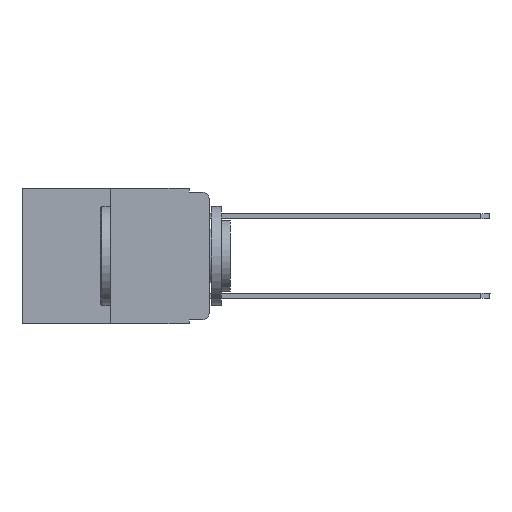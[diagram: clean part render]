
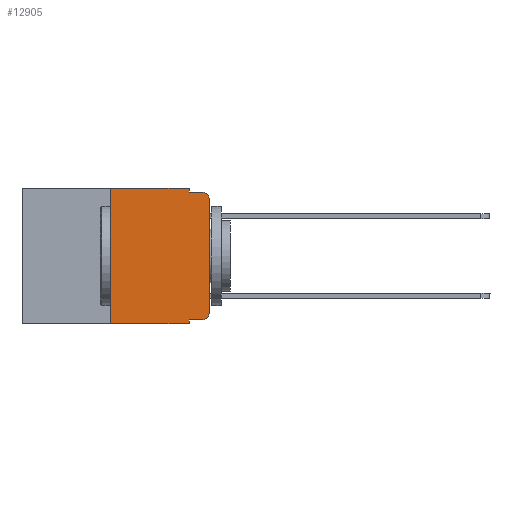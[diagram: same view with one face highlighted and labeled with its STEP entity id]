
A CAD part, left-side view. The second image highlights one B-rep face of the part: STEP entity #12905.
In plain terms, the highlighted planar face has unit normal (-1, 0, 0).
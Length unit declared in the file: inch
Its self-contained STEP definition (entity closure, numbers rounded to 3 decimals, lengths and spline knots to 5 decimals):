
#204 = EDGE_CURVE ( 'NONE', #982, #920, #10719, .T. ) ;
#290 = EDGE_LOOP ( 'NONE', ( #4359, #3330, #5426, #5136, #3894, #4360, #1406, #1857, #1228, #7725 ) ) ;
#349 = VERTEX_POINT ( 'NONE', #13905 ) ;
#687 = DIRECTION ( 'NONE',  ( 1., 0., 0. ) ) ;
#813 = CARTESIAN_POINT ( 'NONE',  ( 0., 0.25, -0.343 ) ) ;
#920 = VERTEX_POINT ( 'NONE', #3082 ) ;
#922 = CARTESIAN_POINT ( 'NONE',  ( 0., 0.051, -0.01 ) ) ;
#982 = VERTEX_POINT ( 'NONE', #15471 ) ;
#996 = DIRECTION ( 'NONE',  ( 0., -1., 0. ) ) ;
#1006 = AXIS2_PLACEMENT_3D ( 'NONE', #8382, #5728, #10912 ) ;
#1228 = ORIENTED_EDGE ( 'NONE', *, *, #2395, .T. ) ;
#1406 = ORIENTED_EDGE ( 'NONE', *, *, #11812, .T. ) ;
#1734 = VERTEX_POINT ( 'NONE', #813 ) ;
#1857 = ORIENTED_EDGE ( 'NONE', *, *, #8401, .F. ) ;
#1917 = CARTESIAN_POINT ( 'NONE',  ( 0., 0.473, 0. ) ) ;
#2174 = CARTESIAN_POINT ( 'NONE',  ( 0., 0.051, -0.333 ) ) ;
#2182 = VECTOR ( 'NONE', #8756, 39.37008 ) ;
#2395 = EDGE_CURVE ( 'NONE', #9739, #3634, #14970, .T. ) ;
#2434 = DIRECTION ( 'NONE',  ( 0., -1., 0. ) ) ;
#2704 = VECTOR ( 'NONE', #2434, 39.37008 ) ;
#3082 = CARTESIAN_POINT ( 'NONE',  ( 0., 0.02, -0.01 ) ) ;
#3330 = ORIENTED_EDGE ( 'NONE', *, *, #204, .T. ) ;
#3525 = DIRECTION ( 'NONE',  ( 0., 0., -1. ) ) ;
#3634 = VERTEX_POINT ( 'NONE', #9755 ) ;
#3663 = CARTESIAN_POINT ( 'NONE',  ( 0., 0.473, -0.343 ) ) ;
#3700 = VECTOR ( 'NONE', #8622, 39.37008 ) ;
#3894 = ORIENTED_EDGE ( 'NONE', *, *, #5141, .F. ) ;
#4005 = DIRECTION ( 'NONE',  ( 0., 0., 1. ) ) ;
#4032 = VERTEX_POINT ( 'NONE', #10787 ) ;
#4270 = PLANE ( 'NONE',  #15746 ) ;
#4359 = ORIENTED_EDGE ( 'NONE', *, *, #12126, .T. ) ;
#4360 = ORIENTED_EDGE ( 'NONE', *, *, #16008, .F. ) ;
#4501 = VERTEX_POINT ( 'NONE', #8149 ) ;
#4517 = DIRECTION ( 'NONE',  ( 0., 0., -1. ) ) ;
#4555 = EDGE_CURVE ( 'NONE', #4501, #4032, #8554, .T. ) ;
#4650 = EDGE_CURVE ( 'NONE', #4032, #920, #6062, .T. ) ;
#4674 = DIRECTION ( 'NONE',  ( 0., 0., -1. ) ) ;
#5136 = ORIENTED_EDGE ( 'NONE', *, *, #4555, .F. ) ;
#5141 = EDGE_CURVE ( 'NONE', #5950, #4501, #9904, .T. ) ;
#5426 = ORIENTED_EDGE ( 'NONE', *, *, #4650, .F. ) ;
#5534 = VECTOR ( 'NONE', #10733, 39.37008 ) ;
#5728 = DIRECTION ( 'NONE',  ( -1., 0., 0. ) ) ;
#5835 = CARTESIAN_POINT ( 'NONE',  ( 0., 0.051, 0. ) ) ;
#5950 = VERTEX_POINT ( 'NONE', #14856 ) ;
#6062 = LINE ( 'NONE', #922, #7103 ) ;
#6280 = VECTOR ( 'NONE', #3525, 39.37008 ) ;
#6657 = CARTESIAN_POINT ( 'NONE',  ( 0., 0.051, -0.333 ) ) ;
#6950 = CARTESIAN_POINT ( 'NONE',  ( 0., 0., 0. ) ) ;
#7103 = VECTOR ( 'NONE', #996, 39.37008 ) ;
#7486 = CARTESIAN_POINT ( 'NONE',  ( 0., 0.051, -0.343 ) ) ;
#7725 = ORIENTED_EDGE ( 'NONE', *, *, #8850, .T. ) ;
#8149 = CARTESIAN_POINT ( 'NONE',  ( 0., 0.051, 0. ) ) ;
#8364 = LINE ( 'NONE', #6950, #5534 ) ;
#8382 = CARTESIAN_POINT ( 'NONE',  ( 0., 0.02, -0.313 ) ) ;
#8401 = EDGE_CURVE ( 'NONE', #9739, #15858, #12327, .T. ) ;
#8454 = DIRECTION ( 'NONE',  ( -1., 0., 0. ) ) ;
#8554 = LINE ( 'NONE', #10922, #6280 ) ;
#8622 = DIRECTION ( 'NONE',  ( 0., -1., 0. ) ) ;
#8756 = DIRECTION ( 'NONE',  ( 0., -1., 0. ) ) ;
#8850 = EDGE_CURVE ( 'NONE', #3634, #349, #15209, .T. ) ;
#9042 = VECTOR ( 'NONE', #4005, 39.37008 ) ;
#9117 = LINE ( 'NONE', #12723, #9042 ) ;
#9739 = VERTEX_POINT ( 'NONE', #6657 ) ;
#9755 = CARTESIAN_POINT ( 'NONE',  ( 0., 0.02, -0.333 ) ) ;
#9904 = LINE ( 'NONE', #14892, #2704 ) ;
#10010 = LINE ( 'NONE', #3663, #3700 ) ;
#10719 = CIRCLE ( 'NONE', #15426, 0.02 ) ;
#10733 = DIRECTION ( 'NONE',  ( 0., 0., 1. ) ) ;
#10787 = CARTESIAN_POINT ( 'NONE',  ( 0., 0.051, -0.01 ) ) ;
#10912 = DIRECTION ( 'NONE',  ( 0., 0., -1. ) ) ;
#10922 = CARTESIAN_POINT ( 'NONE',  ( 0., 0.051, 0. ) ) ;
#11812 = EDGE_CURVE ( 'NONE', #1734, #15858, #10010, .T. ) ;
#12126 = EDGE_CURVE ( 'NONE', #349, #982, #8364, .T. ) ;
#12327 = LINE ( 'NONE', #5835, #14737 ) ;
#12723 = CARTESIAN_POINT ( 'NONE',  ( 0., 0.25, 0. ) ) ;
#12905 = ADVANCED_FACE ( 'NONE', ( #14360 ), #4270, .F. ) ;
#13905 = CARTESIAN_POINT ( 'NONE',  ( 0., 0., -0.313 ) ) ;
#14360 = FACE_OUTER_BOUND ( 'NONE', #290, .T. ) ;
#14661 = CARTESIAN_POINT ( 'NONE',  ( 0., 0.02, -0.03 ) ) ;
#14737 = VECTOR ( 'NONE', #4674, 39.37008 ) ;
#14750 = DIRECTION ( 'NONE',  ( 0., 0., -1. ) ) ;
#14856 = CARTESIAN_POINT ( 'NONE',  ( 0., 0.25, 0. ) ) ;
#14892 = CARTESIAN_POINT ( 'NONE',  ( 0., 0.473, 0. ) ) ;
#14970 = LINE ( 'NONE', #2174, #2182 ) ;
#15209 = CIRCLE ( 'NONE', #1006, 0.02 ) ;
#15426 = AXIS2_PLACEMENT_3D ( 'NONE', #14661, #8454, #14750 ) ;
#15471 = CARTESIAN_POINT ( 'NONE',  ( 0., 0., -0.03 ) ) ;
#15746 = AXIS2_PLACEMENT_3D ( 'NONE', #1917, #687, #4517 ) ;
#15858 = VERTEX_POINT ( 'NONE', #7486 ) ;
#16008 = EDGE_CURVE ( 'NONE', #1734, #5950, #9117, .T. ) ;
